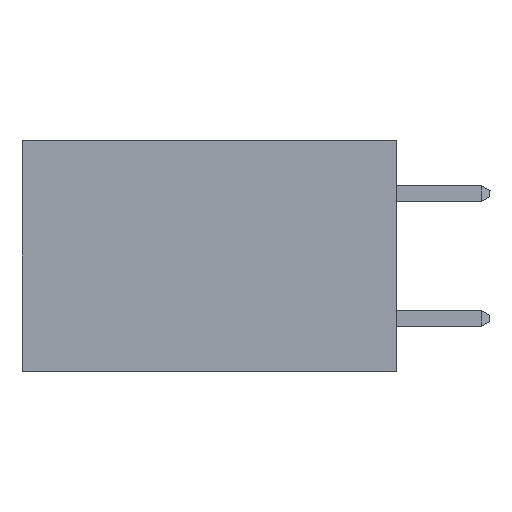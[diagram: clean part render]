
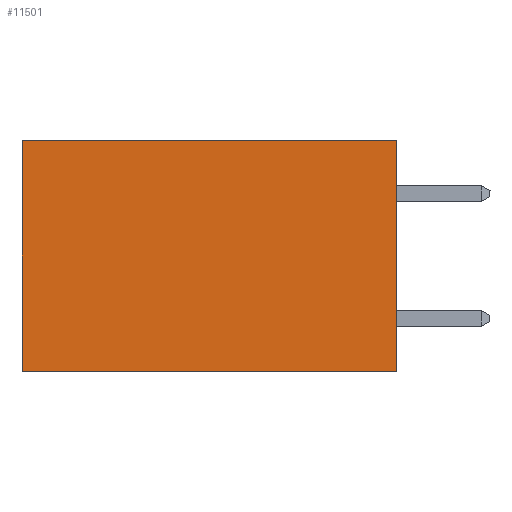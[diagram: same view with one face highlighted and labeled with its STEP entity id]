
A CAD part, left-side view. The second image highlights one B-rep face of the part: STEP entity #11501.
In plain terms, the highlighted planar face has unit normal (-1, 0, 0).
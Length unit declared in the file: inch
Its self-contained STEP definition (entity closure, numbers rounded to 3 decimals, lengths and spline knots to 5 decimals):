
#51 = EDGE_LOOP ( 'NONE', ( #1244, #18413, #13024, #8623 ) ) ;
#1129 = DIRECTION ( 'NONE',  ( 0., 0., -1. ) ) ;
#1155 = DIRECTION ( 'NONE',  ( 1., 0., 0. ) ) ;
#1187 = CARTESIAN_POINT ( 'NONE',  ( 0.298, 0., 0. ) ) ;
#1244 = ORIENTED_EDGE ( 'NONE', *, *, #6987, .T. ) ;
#1312 = PLANE ( 'NONE',  #6721 ) ;
#2189 = LINE ( 'NONE', #17971, #10033 ) ;
#2512 = DIRECTION ( 'NONE',  ( 0., 0., -1. ) ) ;
#3427 = DIRECTION ( 'NONE',  ( 0., 0., -1. ) ) ;
#3507 = CARTESIAN_POINT ( 'NONE',  ( 0.298, 0., 0. ) ) ;
#3820 = LINE ( 'NONE', #3507, #7356 ) ;
#4823 = EDGE_CURVE ( 'NONE', #14877, #7082, #17294, .T. ) ;
#5053 = CARTESIAN_POINT ( 'NONE',  ( 0.298, 0., 0. ) ) ;
#5149 = VECTOR ( 'NONE', #2512, 39.37008 ) ;
#6209 = EDGE_CURVE ( 'NONE', #17070, #18726, #2189, .T. ) ;
#6721 = AXIS2_PLACEMENT_3D ( 'NONE', #1187, #1155, #1129 ) ;
#6987 = EDGE_CURVE ( 'NONE', #7082, #18726, #14394, .T. ) ;
#7082 = VERTEX_POINT ( 'NONE', #10261 ) ;
#7356 = VECTOR ( 'NONE', #3427, 39.37008 ) ;
#8623 = ORIENTED_EDGE ( 'NONE', *, *, #4823, .T. ) ;
#8738 = CARTESIAN_POINT ( 'NONE',  ( 0.298, 0., -0.37 ) ) ;
#9185 = VECTOR ( 'NONE', #14760, 39.37008 ) ;
#10033 = VECTOR ( 'NONE', #18274, 39.37008 ) ;
#10261 = CARTESIAN_POINT ( 'NONE',  ( 0.298, 0.6, 0. ) ) ;
#11220 = EDGE_CURVE ( 'NONE', #14877, #17070, #3820, .T. ) ;
#11501 = ADVANCED_FACE ( 'NONE', ( #18130 ), #1312, .F. ) ;
#13024 = ORIENTED_EDGE ( 'NONE', *, *, #11220, .F. ) ;
#13168 = CARTESIAN_POINT ( 'NONE',  ( 0.298, 0.6, 0. ) ) ;
#14394 = LINE ( 'NONE', #13168, #5149 ) ;
#14760 = DIRECTION ( 'NONE',  ( 0., 1., 0. ) ) ;
#14877 = VERTEX_POINT ( 'NONE', #17103 ) ;
#16346 = CARTESIAN_POINT ( 'NONE',  ( 0.298, 0.6, -0.37 ) ) ;
#17070 = VERTEX_POINT ( 'NONE', #8738 ) ;
#17103 = CARTESIAN_POINT ( 'NONE',  ( 0.298, 0., 0. ) ) ;
#17294 = LINE ( 'NONE', #5053, #9185 ) ;
#17971 = CARTESIAN_POINT ( 'NONE',  ( 0.298, 0., -0.37 ) ) ;
#18130 = FACE_OUTER_BOUND ( 'NONE', #51, .T. ) ;
#18274 = DIRECTION ( 'NONE',  ( 0., 1., 0. ) ) ;
#18413 = ORIENTED_EDGE ( 'NONE', *, *, #6209, .F. ) ;
#18726 = VERTEX_POINT ( 'NONE', #16346 ) ;
